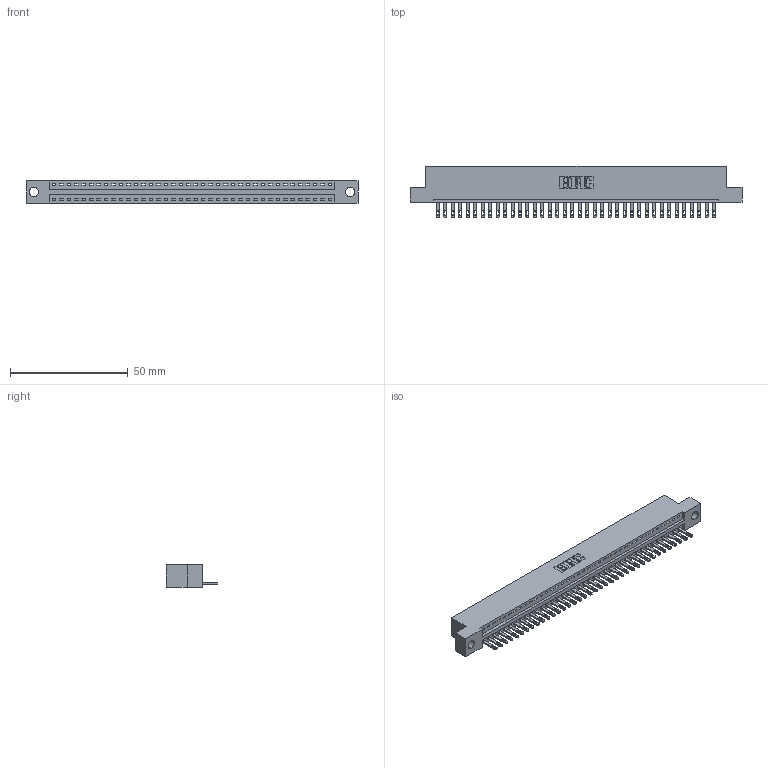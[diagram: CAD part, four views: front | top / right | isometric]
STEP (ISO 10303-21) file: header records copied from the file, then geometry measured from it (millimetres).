
FILE_DESCRIPTION (( 'STEP AP203' ), '1' );
FILE_NAME ('896-038-500-104.STEP', '2021-07-27T20:34:20', ( '' ), ( '' ), 'SwSTEP 2.0', 'SolidWorks 2020', '' );
FILE_SCHEMA (( 'CONFIG_CONTROL_DESIGN' ));
Length unit declared in the file: inch
Products named in the file (3): 896-038-500-104; 345-292-001_345-293-100; 846 Part_Flush Mounting Lugs - 0.156 Dia-TH
Assembly tree (39 placements, depth 2):
  896-038-500-104
    846 Part_Flush Mounting Lugs - 0.156 Dia-TH
    345-292-001_345-293-100  x38
Bounding box: 141.22 x 21.84 x 9.4 mm (x, y, z)
Volume: 13426.4 mm3; surface area: 16631.6 mm2
Topology: 39 solids, 39 shells, 2174 faces, 6713 edges, 4474 vertices
Faces by surface type: plane 1368, cylinder 806
Entity records: 24055 total; most frequent: CARTESIAN_POINT 4130, ORIENTED_EDGE 4102, DIRECTION 3651, EDGE_CURVE 2051, LINE 1763, VECTOR 1763, VERTEX_POINT 1366, AXIS2_PLACEMENT_3D 944
